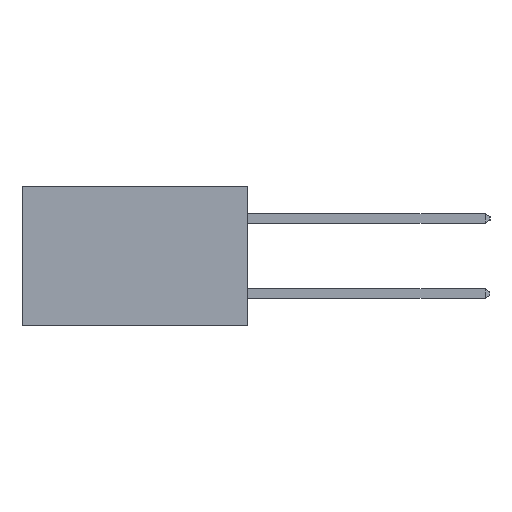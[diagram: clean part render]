
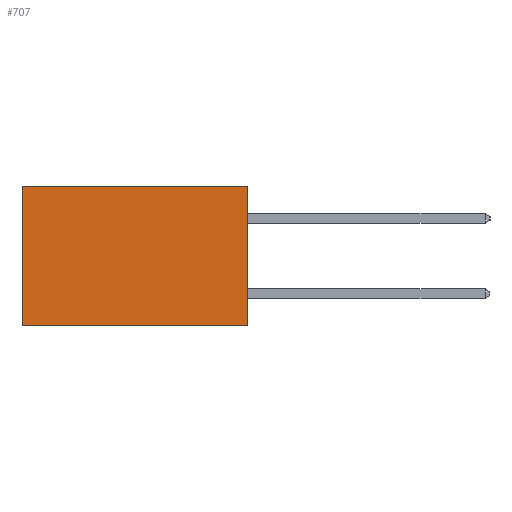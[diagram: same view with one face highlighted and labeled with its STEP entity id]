
A CAD part, left-side view. The second image highlights one B-rep face of the part: STEP entity #707.
In plain terms, the highlighted planar face has unit normal (-1, 0, 0).
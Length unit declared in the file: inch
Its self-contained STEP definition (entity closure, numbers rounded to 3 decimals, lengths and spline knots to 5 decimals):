
#170 = ORIENTED_EDGE ( 'NONE', *, *, #15221, .F. ) ;
#707 = ADVANCED_FACE ( 'NONE', ( #15789 ), #13635, .F. ) ;
#753 = CARTESIAN_POINT ( 'NONE',  ( 0.298, 0., 0. ) ) ;
#1180 = VECTOR ( 'NONE', #10382, 39.37008 ) ;
#2988 = VECTOR ( 'NONE', #4772, 39.37008 ) ;
#3310 = CARTESIAN_POINT ( 'NONE',  ( 0.298, 0.6, 0. ) ) ;
#3359 = CARTESIAN_POINT ( 'NONE',  ( 0.298, 0., 0. ) ) ;
#3393 = LINE ( 'NONE', #10902, #17826 ) ;
#3709 = ORIENTED_EDGE ( 'NONE', *, *, #4073, .T. ) ;
#4073 = EDGE_CURVE ( 'NONE', #17388, #11003, #3393, .T. ) ;
#4772 = DIRECTION ( 'NONE',  ( 0., 1., 0. ) ) ;
#4869 = DIRECTION ( 'NONE',  ( 0., 0., -1. ) ) ;
#7663 = CARTESIAN_POINT ( 'NONE',  ( 0.298, 0., -0.37 ) ) ;
#8008 = CARTESIAN_POINT ( 'NONE',  ( 0.298, 0., 0. ) ) ;
#8183 = VECTOR ( 'NONE', #9093, 39.37008 ) ;
#9093 = DIRECTION ( 'NONE',  ( 0., 0., -1. ) ) ;
#9294 = EDGE_CURVE ( 'NONE', #12697, #10165, #15029, .T. ) ;
#9434 = CARTESIAN_POINT ( 'NONE',  ( 0.298, 0.6, -0.37 ) ) ;
#10165 = VERTEX_POINT ( 'NONE', #9434 ) ;
#10193 = EDGE_LOOP ( 'NONE', ( #16764, #13496, #170, #3709 ) ) ;
#10382 = DIRECTION ( 'NONE',  ( 0., 0., -1. ) ) ;
#10902 = CARTESIAN_POINT ( 'NONE',  ( 0.298, 0., 0. ) ) ;
#11003 = VERTEX_POINT ( 'NONE', #12434 ) ;
#11359 = EDGE_CURVE ( 'NONE', #11003, #10165, #15627, .T. ) ;
#12283 = DIRECTION ( 'NONE',  ( 0., 1., 0. ) ) ;
#12434 = CARTESIAN_POINT ( 'NONE',  ( 0.298, 0.6, 0. ) ) ;
#12483 = AXIS2_PLACEMENT_3D ( 'NONE', #8008, #17377, #4869 ) ;
#12697 = VERTEX_POINT ( 'NONE', #13269 ) ;
#13269 = CARTESIAN_POINT ( 'NONE',  ( 0.298, 0., -0.37 ) ) ;
#13496 = ORIENTED_EDGE ( 'NONE', *, *, #9294, .F. ) ;
#13635 = PLANE ( 'NONE',  #12483 ) ;
#15029 = LINE ( 'NONE', #7663, #2988 ) ;
#15221 = EDGE_CURVE ( 'NONE', #17388, #12697, #15527, .T. ) ;
#15527 = LINE ( 'NONE', #3359, #8183 ) ;
#15627 = LINE ( 'NONE', #3310, #1180 ) ;
#15789 = FACE_OUTER_BOUND ( 'NONE', #10193, .T. ) ;
#16764 = ORIENTED_EDGE ( 'NONE', *, *, #11359, .T. ) ;
#17377 = DIRECTION ( 'NONE',  ( 1., 0., 0. ) ) ;
#17388 = VERTEX_POINT ( 'NONE', #753 ) ;
#17826 = VECTOR ( 'NONE', #12283, 39.37008 ) ;
